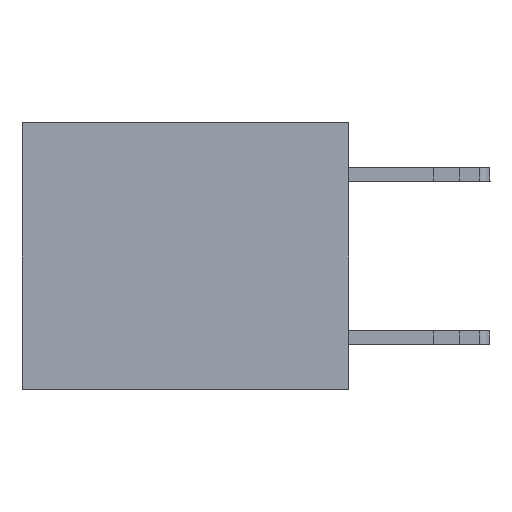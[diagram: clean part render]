
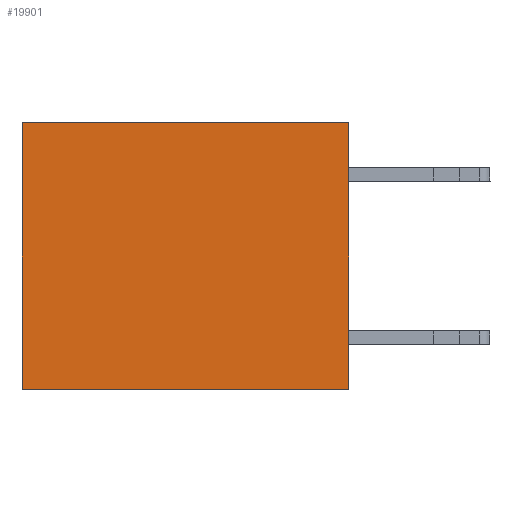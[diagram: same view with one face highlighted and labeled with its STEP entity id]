
A CAD part, left-side view. The second image highlights one B-rep face of the part: STEP entity #19901.
In plain terms, the highlighted planar face has unit normal (-1, 0, 0).
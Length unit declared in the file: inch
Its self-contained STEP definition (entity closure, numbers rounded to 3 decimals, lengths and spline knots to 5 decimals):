
#598 = DIRECTION ( 'NONE',  ( 0., 0., -1. ) ) ;
#1387 = ORIENTED_EDGE ( 'NONE', *, *, #8886, .F. ) ;
#1416 = LINE ( 'NONE', #14949, #19833 ) ;
#2593 = CARTESIAN_POINT ( 'NONE',  ( 0.3165, 0., -0.49 ) ) ;
#3336 = CARTESIAN_POINT ( 'NONE',  ( 0.3165, 0.6, 0. ) ) ;
#4723 = CARTESIAN_POINT ( 'NONE',  ( 0.3165, 0., 0. ) ) ;
#4923 = VECTOR ( 'NONE', #24908, 39.37008 ) ;
#5078 = ORIENTED_EDGE ( 'NONE', *, *, #7800, .T. ) ;
#5230 = CARTESIAN_POINT ( 'NONE',  ( 0.3165, 0.6, -0.49 ) ) ;
#5725 = EDGE_CURVE ( 'NONE', #8817, #5916, #12786, .T. ) ;
#5916 = VERTEX_POINT ( 'NONE', #5230 ) ;
#6849 = AXIS2_PLACEMENT_3D ( 'NONE', #2593, #8877, #598 ) ;
#7126 = ORIENTED_EDGE ( 'NONE', *, *, #5725, .F. ) ;
#7671 = EDGE_CURVE ( 'NONE', #23041, #5916, #9316, .T. ) ;
#7800 = EDGE_CURVE ( 'NONE', #15130, #23041, #1416, .T. ) ;
#8817 = VERTEX_POINT ( 'NONE', #16230 ) ;
#8877 = DIRECTION ( 'NONE',  ( 1., 0., 0. ) ) ;
#8886 = EDGE_CURVE ( 'NONE', #15130, #8817, #15466, .T. ) ;
#9031 = VECTOR ( 'NONE', #18412, 39.37008 ) ;
#9316 = LINE ( 'NONE', #10207, #9031 ) ;
#10114 = CARTESIAN_POINT ( 'NONE',  ( 0.3165, 0., -0.49 ) ) ;
#10207 = CARTESIAN_POINT ( 'NONE',  ( 0.3165, 0.6, -0.49 ) ) ;
#11707 = EDGE_LOOP ( 'NONE', ( #26028, #7126, #1387, #5078 ) ) ;
#12208 = CARTESIAN_POINT ( 'NONE',  ( 0.3165, 0., -0.49 ) ) ;
#12786 = LINE ( 'NONE', #12208, #4923 ) ;
#14949 = CARTESIAN_POINT ( 'NONE',  ( 0.3165, 0., 0. ) ) ;
#15130 = VERTEX_POINT ( 'NONE', #4723 ) ;
#15466 = LINE ( 'NONE', #10114, #18084 ) ;
#16230 = CARTESIAN_POINT ( 'NONE',  ( 0.3165, 0., -0.49 ) ) ;
#16872 = DIRECTION ( 'NONE',  ( 0., 1., 0. ) ) ;
#17397 = FACE_OUTER_BOUND ( 'NONE', #11707, .T. ) ;
#18084 = VECTOR ( 'NONE', #24835, 39.37008 ) ;
#18412 = DIRECTION ( 'NONE',  ( 0., 0., -1. ) ) ;
#19833 = VECTOR ( 'NONE', #16872, 39.37008 ) ;
#19901 = ADVANCED_FACE ( 'NONE', ( #17397 ), #25630, .F. ) ;
#23041 = VERTEX_POINT ( 'NONE', #3336 ) ;
#24835 = DIRECTION ( 'NONE',  ( 0., 0., -1. ) ) ;
#24908 = DIRECTION ( 'NONE',  ( 0., 1., 0. ) ) ;
#25630 = PLANE ( 'NONE',  #6849 ) ;
#26028 = ORIENTED_EDGE ( 'NONE', *, *, #7671, .T. ) ;
